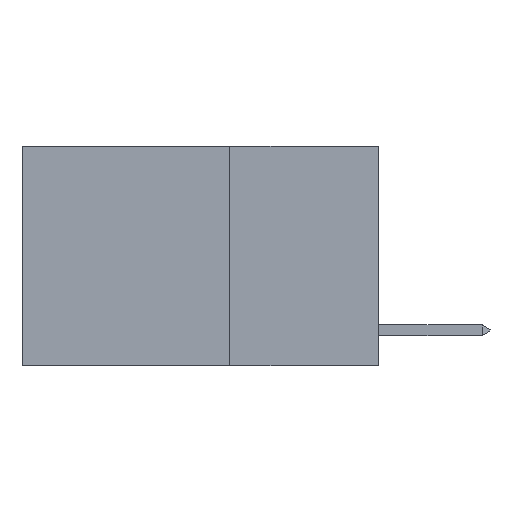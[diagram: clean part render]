
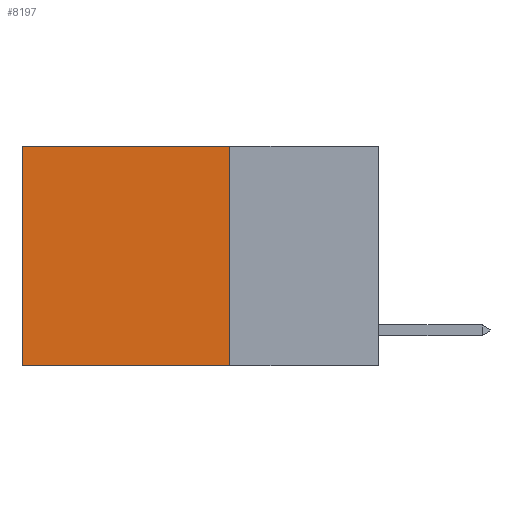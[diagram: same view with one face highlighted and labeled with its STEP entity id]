
A CAD part, left-side view. The second image highlights one B-rep face of the part: STEP entity #8197.
In plain terms, the highlighted planar face has unit normal (-1, 0, 0).
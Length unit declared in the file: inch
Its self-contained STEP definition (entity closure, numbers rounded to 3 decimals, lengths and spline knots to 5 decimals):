
#532 = VECTOR ( 'NONE', #4109, 39.37008 ) ;
#629 = DIRECTION ( 'NONE',  ( 0., 0., -1. ) ) ;
#1087 = EDGE_CURVE ( 'NONE', #8320, #7552, #6668, .T. ) ;
#1913 = DIRECTION ( 'NONE',  ( 0., 0., -1. ) ) ;
#2247 = CARTESIAN_POINT ( 'NONE',  ( 0.2625, 0.25, 0. ) ) ;
#2387 = DIRECTION ( 'NONE',  ( 0., 0., -1. ) ) ;
#2528 = EDGE_CURVE ( 'NONE', #8995, #8792, #3794, .T. ) ;
#2705 = LINE ( 'NONE', #3537, #8059 ) ;
#3537 = CARTESIAN_POINT ( 'NONE',  ( 0.2625, 0.6, 0. ) ) ;
#3701 = LINE ( 'NONE', #2247, #5587 ) ;
#3761 = FACE_OUTER_BOUND ( 'NONE', #6841, .T. ) ;
#3794 = LINE ( 'NONE', #5316, #5445 ) ;
#4109 = DIRECTION ( 'NONE',  ( 0., 1., 0. ) ) ;
#4131 = CARTESIAN_POINT ( 'NONE',  ( 0.2625, 0.25, 0. ) ) ;
#4366 = EDGE_CURVE ( 'NONE', #7552, #8792, #2705, .T. ) ;
#4641 = EDGE_CURVE ( 'NONE', #8320, #8995, #3701, .T. ) ;
#4799 = PLANE ( 'NONE',  #8518 ) ;
#5231 = DIRECTION ( 'NONE',  ( 0., 1., 0. ) ) ;
#5316 = CARTESIAN_POINT ( 'NONE',  ( 0.2625, 0.25, -0.37 ) ) ;
#5445 = VECTOR ( 'NONE', #5231, 39.37008 ) ;
#5587 = VECTOR ( 'NONE', #629, 39.37008 ) ;
#5748 = ORIENTED_EDGE ( 'NONE', *, *, #1087, .T. ) ;
#5750 = ORIENTED_EDGE ( 'NONE', *, *, #4641, .F. ) ;
#6371 = CARTESIAN_POINT ( 'NONE',  ( 0.2625, 0.25, 0. ) ) ;
#6558 = CARTESIAN_POINT ( 'NONE',  ( 0.2625, 0.25, 0. ) ) ;
#6668 = LINE ( 'NONE', #4131, #532 ) ;
#6676 = CARTESIAN_POINT ( 'NONE',  ( 0.2625, 0.25, -0.37 ) ) ;
#6841 = EDGE_LOOP ( 'NONE', ( #8813, #7662, #5750, #5748 ) ) ;
#7152 = DIRECTION ( 'NONE',  ( 1., 0., 0. ) ) ;
#7552 = VERTEX_POINT ( 'NONE', #10173 ) ;
#7662 = ORIENTED_EDGE ( 'NONE', *, *, #2528, .F. ) ;
#8059 = VECTOR ( 'NONE', #1913, 39.37008 ) ;
#8197 = ADVANCED_FACE ( 'NONE', ( #3761 ), #4799, .F. ) ;
#8320 = VERTEX_POINT ( 'NONE', #6558 ) ;
#8518 = AXIS2_PLACEMENT_3D ( 'NONE', #6371, #7152, #2387 ) ;
#8667 = CARTESIAN_POINT ( 'NONE',  ( 0.2625, 0.6, -0.37 ) ) ;
#8792 = VERTEX_POINT ( 'NONE', #8667 ) ;
#8813 = ORIENTED_EDGE ( 'NONE', *, *, #4366, .T. ) ;
#8995 = VERTEX_POINT ( 'NONE', #6676 ) ;
#10173 = CARTESIAN_POINT ( 'NONE',  ( 0.2625, 0.6, 0. ) ) ;
